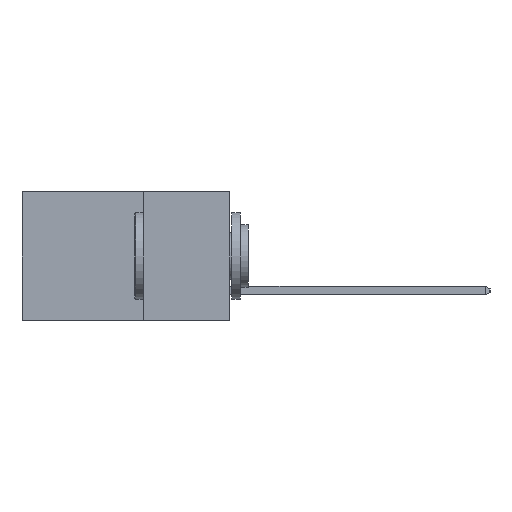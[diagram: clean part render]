
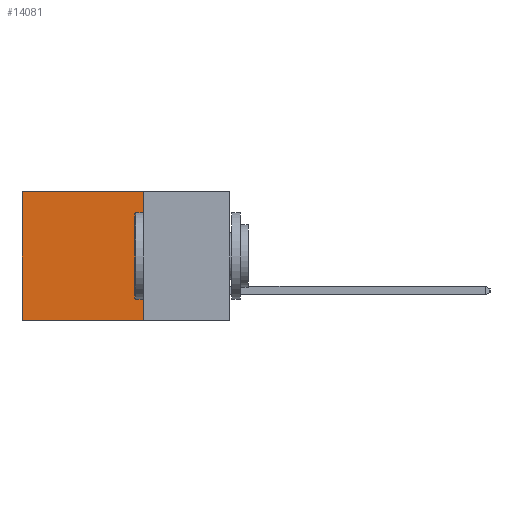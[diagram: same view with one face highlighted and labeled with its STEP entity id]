
A CAD part, left-side view. The second image highlights one B-rep face of the part: STEP entity #14081.
In plain terms, the highlighted planar face has unit normal (-1, 0, 0).
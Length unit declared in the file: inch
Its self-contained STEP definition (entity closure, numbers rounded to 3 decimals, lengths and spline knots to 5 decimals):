
#677 = ORIENTED_EDGE ( 'NONE', *, *, #1900, .F. ) ;
#866 = VERTEX_POINT ( 'NONE', #9122 ) ;
#886 = LINE ( 'NONE', #4723, #20323 ) ;
#1900 = EDGE_CURVE ( 'NONE', #9524, #866, #886, .T. ) ;
#2317 = DIRECTION ( 'NONE',  ( 0., 1., 0. ) ) ;
#2408 = EDGE_CURVE ( 'NONE', #3817, #9524, #15496, .T. ) ;
#2656 = VERTEX_POINT ( 'NONE', #11345 ) ;
#3485 = VECTOR ( 'NONE', #6073, 39.37008 ) ;
#3817 = VERTEX_POINT ( 'NONE', #18628 ) ;
#3937 = LINE ( 'NONE', #6590, #4431 ) ;
#4431 = VECTOR ( 'NONE', #6700, 39.37008 ) ;
#4723 = CARTESIAN_POINT ( 'NONE',  ( 0.2615, 0.25, -0.37 ) ) ;
#5329 = DIRECTION ( 'NONE',  ( 0., 1., 0. ) ) ;
#5857 = CARTESIAN_POINT ( 'NONE',  ( 0.2615, 0.25, 0. ) ) ;
#6050 = CARTESIAN_POINT ( 'NONE',  ( 0.2615, 0.25, -0.37 ) ) ;
#6073 = DIRECTION ( 'NONE',  ( 0., 0., -1. ) ) ;
#6590 = CARTESIAN_POINT ( 'NONE',  ( 0.2615, 0.6, -0.37 ) ) ;
#6700 = DIRECTION ( 'NONE',  ( 0., 0., -1. ) ) ;
#6907 = ORIENTED_EDGE ( 'NONE', *, *, #7611, .T. ) ;
#7611 = EDGE_CURVE ( 'NONE', #2656, #866, #3937, .T. ) ;
#8404 = FACE_OUTER_BOUND ( 'NONE', #18073, .T. ) ;
#9122 = CARTESIAN_POINT ( 'NONE',  ( 0.2615, 0.6, -0.37 ) ) ;
#9524 = VERTEX_POINT ( 'NONE', #14991 ) ;
#9809 = EDGE_CURVE ( 'NONE', #3817, #2656, #20245, .T. ) ;
#10810 = DIRECTION ( 'NONE',  ( 0., 0., -1. ) ) ;
#11345 = CARTESIAN_POINT ( 'NONE',  ( 0.2615, 0.6, 0. ) ) ;
#14081 = ADVANCED_FACE ( 'NONE', ( #8404 ), #18655, .F. ) ;
#14991 = CARTESIAN_POINT ( 'NONE',  ( 0.2615, 0.25, -0.37 ) ) ;
#15155 = VECTOR ( 'NONE', #5329, 39.37008 ) ;
#15496 = LINE ( 'NONE', #6050, #3485 ) ;
#16489 = ORIENTED_EDGE ( 'NONE', *, *, #2408, .F. ) ;
#16783 = ORIENTED_EDGE ( 'NONE', *, *, #9809, .T. ) ;
#17189 = CARTESIAN_POINT ( 'NONE',  ( 0.2615, 0.25, -0.37 ) ) ;
#18073 = EDGE_LOOP ( 'NONE', ( #6907, #677, #16489, #16783 ) ) ;
#18482 = AXIS2_PLACEMENT_3D ( 'NONE', #17189, #20200, #10810 ) ;
#18628 = CARTESIAN_POINT ( 'NONE',  ( 0.2615, 0.25, 0. ) ) ;
#18655 = PLANE ( 'NONE',  #18482 ) ;
#20200 = DIRECTION ( 'NONE',  ( 1., 0., 0. ) ) ;
#20245 = LINE ( 'NONE', #5857, #15155 ) ;
#20323 = VECTOR ( 'NONE', #2317, 39.37008 ) ;
